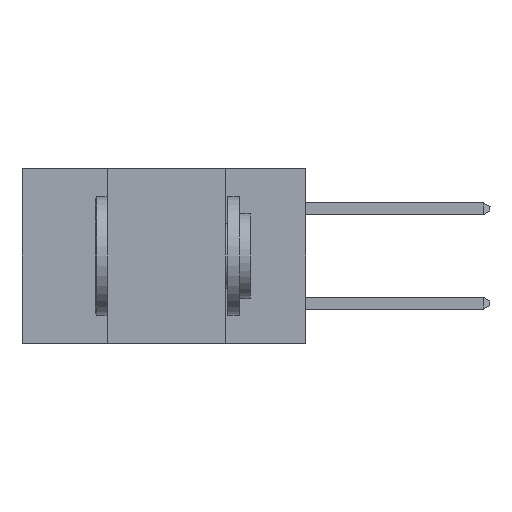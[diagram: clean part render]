
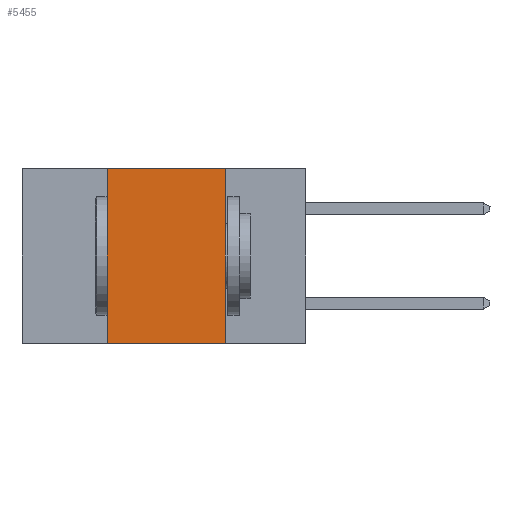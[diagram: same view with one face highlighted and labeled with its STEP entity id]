
A CAD part, left-side view. The second image highlights one B-rep face of the part: STEP entity #5455.
In plain terms, the highlighted planar face has unit normal (-1, 0, 0).
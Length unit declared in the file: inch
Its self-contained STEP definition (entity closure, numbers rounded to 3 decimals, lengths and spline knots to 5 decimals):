
#348 = VERTEX_POINT ( 'NONE', #9004 ) ;
#1135 = CARTESIAN_POINT ( 'NONE',  ( 0., 0.6, 0. ) ) ;
#1297 = DIRECTION ( 'NONE',  ( 1., 0., 0. ) ) ;
#1399 = DIRECTION ( 'NONE',  ( 0., 0., 1. ) ) ;
#1670 = LINE ( 'NONE', #11682, #5954 ) ;
#1990 = LINE ( 'NONE', #20950, #4555 ) ;
#2299 = EDGE_LOOP ( 'NONE', ( #18471, #19721, #8054, #18985 ) ) ;
#2436 = DIRECTION ( 'NONE',  ( 0., -1., 0. ) ) ;
#3010 = DIRECTION ( 'NONE',  ( 0., 0., -1. ) ) ;
#3192 = LINE ( 'NONE', #19747, #14027 ) ;
#4240 = VERTEX_POINT ( 'NONE', #23664 ) ;
#4277 = DIRECTION ( 'NONE',  ( 0., 0., -1. ) ) ;
#4555 = VECTOR ( 'NONE', #9863, 39.37008 ) ;
#5455 = ADVANCED_FACE ( 'NONE', ( #9396 ), #21251, .F. ) ;
#5954 = VECTOR ( 'NONE', #4277, 39.37008 ) ;
#8054 = ORIENTED_EDGE ( 'NONE', *, *, #8075, .F. ) ;
#8075 = EDGE_CURVE ( 'NONE', #10929, #4240, #3192, .T. ) ;
#9004 = CARTESIAN_POINT ( 'NONE',  ( 0., 0.17, 0. ) ) ;
#9396 = FACE_OUTER_BOUND ( 'NONE', #2299, .T. ) ;
#9714 = EDGE_CURVE ( 'NONE', #348, #20706, #1670, .T. ) ;
#9863 = DIRECTION ( 'NONE',  ( 0., -1., 0. ) ) ;
#10929 = VERTEX_POINT ( 'NONE', #17845 ) ;
#11682 = CARTESIAN_POINT ( 'NONE',  ( 0., 0.17, 0. ) ) ;
#11935 = VECTOR ( 'NONE', #2436, 39.37008 ) ;
#12728 = AXIS2_PLACEMENT_3D ( 'NONE', #1135, #1297, #3010 ) ;
#13347 = CARTESIAN_POINT ( 'NONE',  ( 0., 0.6, -0.37 ) ) ;
#14027 = VECTOR ( 'NONE', #1399, 39.37008 ) ;
#14182 = EDGE_CURVE ( 'NONE', #10929, #20706, #21365, .T. ) ;
#16371 = CARTESIAN_POINT ( 'NONE',  ( 0., 0.17, -0.37 ) ) ;
#17845 = CARTESIAN_POINT ( 'NONE',  ( 0., 0.42, -0.37 ) ) ;
#18471 = ORIENTED_EDGE ( 'NONE', *, *, #9714, .F. ) ;
#18985 = ORIENTED_EDGE ( 'NONE', *, *, #14182, .T. ) ;
#19721 = ORIENTED_EDGE ( 'NONE', *, *, #20930, .F. ) ;
#19747 = CARTESIAN_POINT ( 'NONE',  ( 0., 0.42, 0. ) ) ;
#20706 = VERTEX_POINT ( 'NONE', #16371 ) ;
#20930 = EDGE_CURVE ( 'NONE', #4240, #348, #1990, .T. ) ;
#20950 = CARTESIAN_POINT ( 'NONE',  ( 0., 0.6, 0. ) ) ;
#21251 = PLANE ( 'NONE',  #12728 ) ;
#21365 = LINE ( 'NONE', #13347, #11935 ) ;
#23664 = CARTESIAN_POINT ( 'NONE',  ( 0., 0.42, 0. ) ) ;
